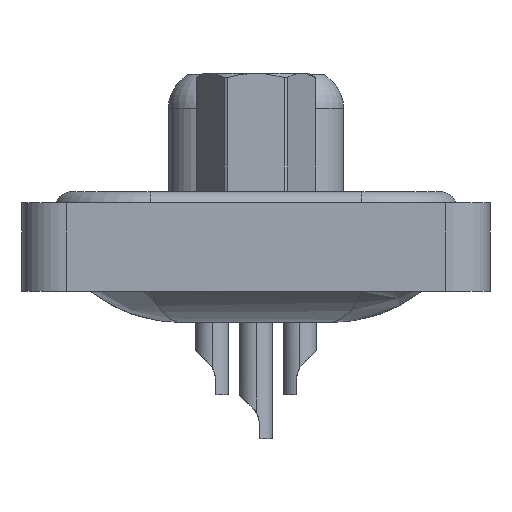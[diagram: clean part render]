
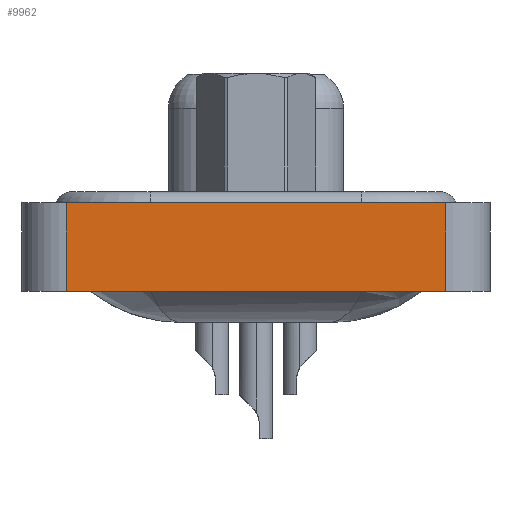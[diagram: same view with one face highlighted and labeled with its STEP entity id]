
A CAD part, left-side view. The second image highlights one B-rep face of the part: STEP entity #9962.
In plain terms, the highlighted planar face has unit normal (-1, 0, 0).
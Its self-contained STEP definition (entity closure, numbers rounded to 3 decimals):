
#167 = VECTOR ( 'NONE', #23857, 1000. ) ;
#1694 = CARTESIAN_POINT ( 'NONE',  ( -7.285, 8.55, -3.6 ) ) ;
#3342 = CARTESIAN_POINT ( 'NONE',  ( -7.285, -8.55, -3.6 ) ) ;
#4029 = VECTOR ( 'NONE', #16022, 1000. ) ;
#5709 = DIRECTION ( 'NONE',  ( -1., 0., 0. ) ) ;
#7435 = AXIS2_PLACEMENT_3D ( 'NONE', #20024, #5709, #22436 ) ;
#8117 = LINE ( 'NONE', #1694, #4029 ) ;
#9008 = EDGE_LOOP ( 'NONE', ( #16286, #14816, #11529, #17247 ) ) ;
#9045 = DIRECTION ( 'NONE',  ( 0., -1., 0. ) ) ;
#9545 = EDGE_CURVE ( 'NONE', #10487, #15024, #28132, .T. ) ;
#9962 = ADVANCED_FACE ( 'NONE', ( #23222 ), #10376, .T. ) ;
#10376 = PLANE ( 'NONE',  #7435 ) ;
#10426 = CARTESIAN_POINT ( 'NONE',  ( -7.285, -8.55, 0.4 ) ) ;
#10487 = VERTEX_POINT ( 'NONE', #18079 ) ;
#10766 = VECTOR ( 'NONE', #16304, 1000. ) ;
#10849 = EDGE_CURVE ( 'NONE', #25624, #15024, #29881, .T. ) ;
#11369 = EDGE_CURVE ( 'NONE', #25533, #10487, #8117, .T. ) ;
#11529 = ORIENTED_EDGE ( 'NONE', *, *, #11369, .F. ) ;
#13214 = EDGE_CURVE ( 'NONE', #25533, #25624, #25711, .T. ) ;
#14816 = ORIENTED_EDGE ( 'NONE', *, *, #9545, .F. ) ;
#15024 = VERTEX_POINT ( 'NONE', #10426 ) ;
#16022 = DIRECTION ( 'NONE',  ( 0., 0., 1. ) ) ;
#16286 = ORIENTED_EDGE ( 'NONE', *, *, #10849, .T. ) ;
#16304 = DIRECTION ( 'NONE',  ( 0., 0., 1. ) ) ;
#17247 = ORIENTED_EDGE ( 'NONE', *, *, #13214, .T. ) ;
#18079 = CARTESIAN_POINT ( 'NONE',  ( -7.285, 8.55, 0.4 ) ) ;
#20024 = CARTESIAN_POINT ( 'NONE',  ( -7.285, -8.55, -3.6 ) ) ;
#22215 = CARTESIAN_POINT ( 'NONE',  ( -7.285, 8.55, -3.6 ) ) ;
#22436 = DIRECTION ( 'NONE',  ( 0., 0., 1. ) ) ;
#23222 = FACE_OUTER_BOUND ( 'NONE', #9008, .T. ) ;
#23418 = CARTESIAN_POINT ( 'NONE',  ( -7.285, -8.55, 0.4 ) ) ;
#23857 = DIRECTION ( 'NONE',  ( 0., -1., 0. ) ) ;
#25533 = VERTEX_POINT ( 'NONE', #22215 ) ;
#25624 = VERTEX_POINT ( 'NONE', #3342 ) ;
#25711 = LINE ( 'NONE', #26313, #167 ) ;
#26313 = CARTESIAN_POINT ( 'NONE',  ( -7.285, -8.55, -3.6 ) ) ;
#27391 = VECTOR ( 'NONE', #9045, 1000. ) ;
#28132 = LINE ( 'NONE', #23418, #27391 ) ;
#29881 = LINE ( 'NONE', #30667, #10766 ) ;
#30667 = CARTESIAN_POINT ( 'NONE',  ( -7.285, -8.55, -3.6 ) ) ;
